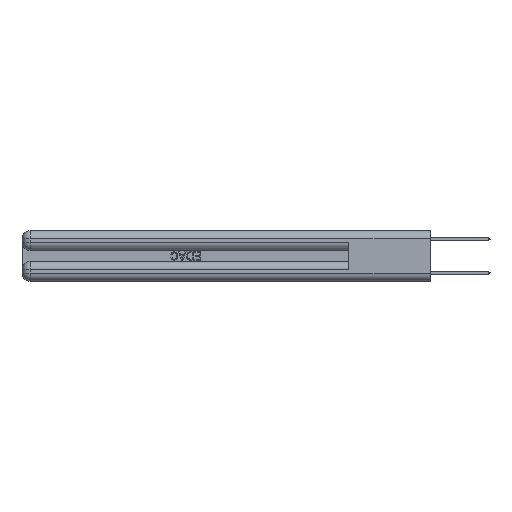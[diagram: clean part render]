
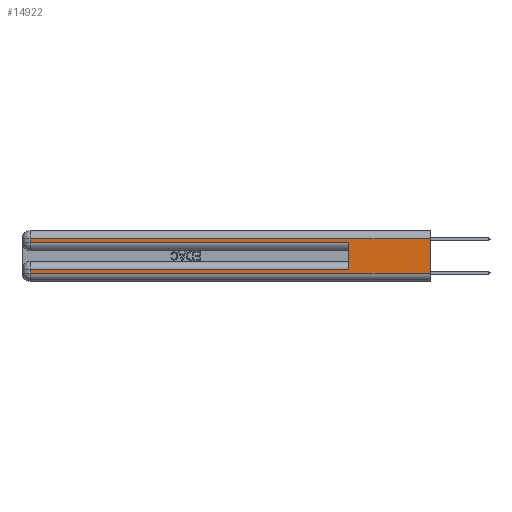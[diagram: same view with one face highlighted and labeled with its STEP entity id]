
A CAD part, left-side view. The second image highlights one B-rep face of the part: STEP entity #14922.
In plain terms, the highlighted planar face has unit normal (-1, 0, 0).
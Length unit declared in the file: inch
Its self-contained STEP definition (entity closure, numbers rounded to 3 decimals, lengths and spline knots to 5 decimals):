
#480 = ORIENTED_EDGE ( 'NONE', *, *, #24795, .T. ) ;
#702 = ORIENTED_EDGE ( 'NONE', *, *, #8647, .T. ) ;
#1435 = DIRECTION ( 'NONE',  ( 0., 1., 0. ) ) ;
#3429 = VERTEX_POINT ( 'NONE', #32313 ) ;
#3581 = CARTESIAN_POINT ( 'NONE',  ( 0., 2.94, 0.37 ) ) ;
#3806 = LINE ( 'NONE', #6514, #34058 ) ;
#4028 = CARTESIAN_POINT ( 'NONE',  ( 0., 0., 0.31 ) ) ;
#4071 = VERTEX_POINT ( 'NONE', #11826 ) ;
#5299 = ORIENTED_EDGE ( 'NONE', *, *, #25777, .T. ) ;
#6076 = DIRECTION ( 'NONE',  ( 0., 1., 0. ) ) ;
#6514 = CARTESIAN_POINT ( 'NONE',  ( 0., 0., 0.31 ) ) ;
#6981 = EDGE_CURVE ( 'NONE', #33625, #22369, #18577, .T. ) ;
#7657 = DIRECTION ( 'NONE',  ( 0., 0., -1. ) ) ;
#7839 = DIRECTION ( 'NONE',  ( 1., 0., 0. ) ) ;
#8647 = EDGE_CURVE ( 'NONE', #9913, #4071, #20886, .T. ) ;
#9348 = VECTOR ( 'NONE', #34264, 39.37008 ) ;
#9739 = VECTOR ( 'NONE', #25607, 39.37008 ) ;
#9913 = VERTEX_POINT ( 'NONE', #29200 ) ;
#10016 = VECTOR ( 'NONE', #19026, 39.37008 ) ;
#10143 = CARTESIAN_POINT ( 'NONE',  ( 0., 0., 0.37 ) ) ;
#10314 = LINE ( 'NONE', #10143, #18747 ) ;
#10668 = PLANE ( 'NONE',  #14959 ) ;
#11561 = LINE ( 'NONE', #25958, #9739 ) ;
#11826 = CARTESIAN_POINT ( 'NONE',  ( 0., 2.94, 0.285 ) ) ;
#11935 = EDGE_CURVE ( 'NONE', #3429, #12442, #11561, .T. ) ;
#12418 = LINE ( 'NONE', #3581, #9348 ) ;
#12442 = VERTEX_POINT ( 'NONE', #25743 ) ;
#12603 = DIRECTION ( 'NONE',  ( 0., 0., -1. ) ) ;
#14922 = ADVANCED_FACE ( 'NONE', ( #33202 ), #10668, .F. ) ;
#14959 = AXIS2_PLACEMENT_3D ( 'NONE', #18651, #7839, #7657 ) ;
#15290 = VERTEX_POINT ( 'NONE', #4028 ) ;
#18577 = LINE ( 'NONE', #32306, #18715 ) ;
#18651 = CARTESIAN_POINT ( 'NONE',  ( 0., 0., 0.37 ) ) ;
#18715 = VECTOR ( 'NONE', #34315, 39.37008 ) ;
#18747 = VECTOR ( 'NONE', #29594, 39.37008 ) ;
#19026 = DIRECTION ( 'NONE',  ( 0., -1., 0. ) ) ;
#19566 = CARTESIAN_POINT ( 'NONE',  ( 0., 0., 0.285 ) ) ;
#19771 = LINE ( 'NONE', #30771, #35199 ) ;
#20459 = EDGE_LOOP ( 'NONE', ( #29221, #26280, #702, #26641, #27130, #480, #5299, #34417 ) ) ;
#20886 = LINE ( 'NONE', #23769, #29168 ) ;
#21086 = VERTEX_POINT ( 'NONE', #28396 ) ;
#22267 = LINE ( 'NONE', #19566, #10016 ) ;
#22369 = VERTEX_POINT ( 'NONE', #25877 ) ;
#23769 = CARTESIAN_POINT ( 'NONE',  ( 0., 2.94, 0.37 ) ) ;
#24795 = EDGE_CURVE ( 'NONE', #3429, #21086, #19771, .T. ) ;
#25607 = DIRECTION ( 'NONE',  ( 0., 0., 1. ) ) ;
#25743 = CARTESIAN_POINT ( 'NONE',  ( 0., 0.6, 0.285 ) ) ;
#25777 = EDGE_CURVE ( 'NONE', #21086, #33625, #12418, .T. ) ;
#25877 = CARTESIAN_POINT ( 'NONE',  ( 0., 0., 0.06 ) ) ;
#25958 = CARTESIAN_POINT ( 'NONE',  ( 0., 0.6, 0.145 ) ) ;
#26280 = ORIENTED_EDGE ( 'NONE', *, *, #34322, .T. ) ;
#26641 = ORIENTED_EDGE ( 'NONE', *, *, #29488, .T. ) ;
#26805 = CARTESIAN_POINT ( 'NONE',  ( 0., 2.94, 0.06 ) ) ;
#27130 = ORIENTED_EDGE ( 'NONE', *, *, #11935, .F. ) ;
#28396 = CARTESIAN_POINT ( 'NONE',  ( 0., 2.94, 0.085 ) ) ;
#29168 = VECTOR ( 'NONE', #12603, 39.37008 ) ;
#29200 = CARTESIAN_POINT ( 'NONE',  ( 0., 2.94, 0.31 ) ) ;
#29221 = ORIENTED_EDGE ( 'NONE', *, *, #31501, .F. ) ;
#29488 = EDGE_CURVE ( 'NONE', #4071, #12442, #22267, .T. ) ;
#29594 = DIRECTION ( 'NONE',  ( 0., 0., -1. ) ) ;
#30771 = CARTESIAN_POINT ( 'NONE',  ( 0., 0., 0.085 ) ) ;
#31501 = EDGE_CURVE ( 'NONE', #15290, #22369, #10314, .T. ) ;
#32306 = CARTESIAN_POINT ( 'NONE',  ( 0., 0., 0.06 ) ) ;
#32313 = CARTESIAN_POINT ( 'NONE',  ( 0., 0.6, 0.085 ) ) ;
#33202 = FACE_OUTER_BOUND ( 'NONE', #20459, .T. ) ;
#33625 = VERTEX_POINT ( 'NONE', #26805 ) ;
#34058 = VECTOR ( 'NONE', #1435, 39.37008 ) ;
#34264 = DIRECTION ( 'NONE',  ( 0., 0., -1. ) ) ;
#34315 = DIRECTION ( 'NONE',  ( 0., -1., 0. ) ) ;
#34322 = EDGE_CURVE ( 'NONE', #15290, #9913, #3806, .T. ) ;
#34417 = ORIENTED_EDGE ( 'NONE', *, *, #6981, .T. ) ;
#35199 = VECTOR ( 'NONE', #6076, 39.37008 ) ;
